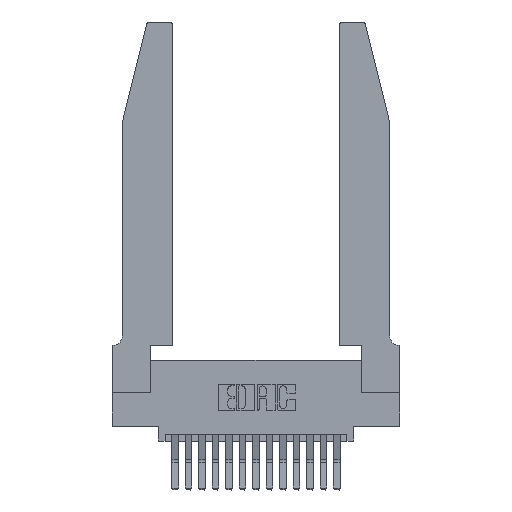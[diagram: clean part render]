
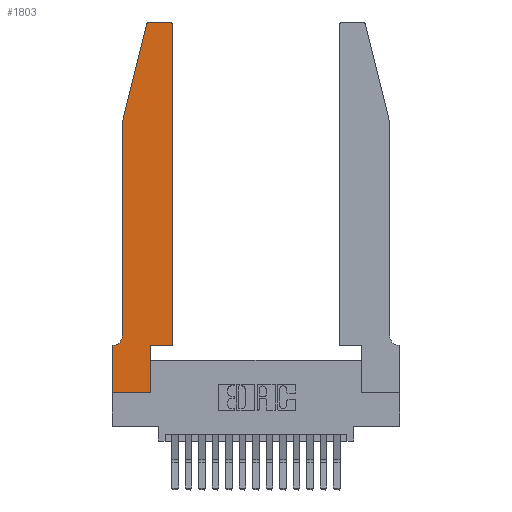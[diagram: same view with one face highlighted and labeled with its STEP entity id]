
A CAD part, top view. The second image highlights one B-rep face of the part: STEP entity #1803.
In plain terms, the highlighted planar face has unit normal (0, 0, 1).
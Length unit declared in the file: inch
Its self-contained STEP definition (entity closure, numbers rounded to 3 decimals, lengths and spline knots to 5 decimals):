
#357 = VERTEX_POINT ( 'NONE', #715 ) ;
#449 = AXIS2_PLACEMENT_3D ( 'NONE', #3735, #16731, #18242 ) ;
#673 = LINE ( 'NONE', #10025, #14673 ) ;
#715 = CARTESIAN_POINT ( 'NONE',  ( 0.2865, 0.35, 0.37 ) ) ;
#806 = CARTESIAN_POINT ( 'NONE',  ( 0.0055, 0.42, 0.37 ) ) ;
#818 = VECTOR ( 'NONE', #17683, 39.37008 ) ;
#869 = VECTOR ( 'NONE', #14858, 39.37008 ) ;
#1104 = ORIENTED_EDGE ( 'NONE', *, *, #1536, .T. ) ;
#1217 = VECTOR ( 'NONE', #18431, 39.37008 ) ;
#1273 = VERTEX_POINT ( 'NONE', #3354 ) ;
#1335 = EDGE_CURVE ( 'NONE', #11629, #10156, #16044, .T. ) ;
#1536 = EDGE_CURVE ( 'NONE', #2989, #9075, #16977, .T. ) ;
#1762 = EDGE_CURVE ( 'NONE', #1273, #7864, #10066, .T. ) ;
#1780 = EDGE_CURVE ( 'NONE', #9075, #6343, #16939, .T. ) ;
#1803 = ADVANCED_FACE ( 'NONE', ( #9216 ), #12288, .T. ) ;
#1937 = EDGE_CURVE ( 'NONE', #10156, #17461, #10199, .T. ) ;
#2416 = AXIS2_PLACEMENT_3D ( 'NONE', #15321, #6591, #6460 ) ;
#2774 = LINE ( 'NONE', #13495, #18003 ) ;
#2815 = DIRECTION ( 'NONE',  ( 1., 0., 0. ) ) ;
#2926 = CIRCLE ( 'NONE', #15723, 0.07 ) ;
#2989 = VERTEX_POINT ( 'NONE', #16043 ) ;
#3165 = CARTESIAN_POINT ( 'NONE',  ( 0.0755, 2., 0.37 ) ) ;
#3354 = CARTESIAN_POINT ( 'NONE',  ( 0.4505, 2.72, 0.37 ) ) ;
#3355 = CARTESIAN_POINT ( 'NONE',  ( 0.0055, 0.35, 0.37 ) ) ;
#3501 = VERTEX_POINT ( 'NONE', #12996 ) ;
#3607 = DIRECTION ( 'NONE',  ( 0., 0., -1. ) ) ;
#3735 = CARTESIAN_POINT ( 'NONE',  ( 0.4205, 2.72, 0.37 ) ) ;
#3738 = LINE ( 'NONE', #7984, #9475 ) ;
#4122 = EDGE_CURVE ( 'NONE', #6117, #2989, #13686, .T. ) ;
#4734 = DIRECTION ( 'NONE',  ( -0.239, -0.971, 0. ) ) ;
#5915 = CARTESIAN_POINT ( 'NONE',  ( 0.0755, 0.42, 0.37 ) ) ;
#6117 = VERTEX_POINT ( 'NONE', #3355 ) ;
#6247 = ORIENTED_EDGE ( 'NONE', *, *, #11947, .T. ) ;
#6343 = VERTEX_POINT ( 'NONE', #10061 ) ;
#6460 = DIRECTION ( 'NONE',  ( 1., 0., 0. ) ) ;
#6463 = AXIS2_PLACEMENT_3D ( 'NONE', #11657, #7205, #2815 ) ;
#6591 = DIRECTION ( 'NONE',  ( 0., 0., 1. ) ) ;
#7061 = ORIENTED_EDGE ( 'NONE', *, *, #7689, .T. ) ;
#7205 = DIRECTION ( 'NONE',  ( 0., 0., 1. ) ) ;
#7267 = CARTESIAN_POINT ( 'NONE',  ( 0.284, 2.75, 0.37 ) ) ;
#7689 = EDGE_CURVE ( 'NONE', #7703, #11629, #12498, .T. ) ;
#7703 = VERTEX_POINT ( 'NONE', #7267 ) ;
#7725 = VECTOR ( 'NONE', #17189, 39.37008 ) ;
#7864 = VERTEX_POINT ( 'NONE', #17652 ) ;
#7879 = EDGE_CURVE ( 'NONE', #6343, #357, #2774, .T. ) ;
#7931 = CARTESIAN_POINT ( 'NONE',  ( 0., 0., 0.37 ) ) ;
#7984 = CARTESIAN_POINT ( 'NONE',  ( 0.4505, 0.35, 0.37 ) ) ;
#8126 = CARTESIAN_POINT ( 'NONE',  ( 0.4505, 0.35, 0.37 ) ) ;
#9005 = CARTESIAN_POINT ( 'NONE',  ( 0., 0., 0.37 ) ) ;
#9075 = VERTEX_POINT ( 'NONE', #13056 ) ;
#9216 = FACE_OUTER_BOUND ( 'NONE', #15425, .T. ) ;
#9310 = ORIENTED_EDGE ( 'NONE', *, *, #16591, .T. ) ;
#9475 = VECTOR ( 'NONE', #16996, 39.37008 ) ;
#10025 = CARTESIAN_POINT ( 'NONE',  ( 0.2605, 2.75, 0.37 ) ) ;
#10061 = CARTESIAN_POINT ( 'NONE',  ( 0.2865, 0., 0.37 ) ) ;
#10066 = CIRCLE ( 'NONE', #449, 0.03 ) ;
#10156 = VERTEX_POINT ( 'NONE', #17405 ) ;
#10199 = LINE ( 'NONE', #14134, #7725 ) ;
#10365 = ORIENTED_EDGE ( 'NONE', *, *, #1762, .T. ) ;
#10880 = VECTOR ( 'NONE', #12409, 39.37008 ) ;
#10912 = ORIENTED_EDGE ( 'NONE', *, *, #1780, .T. ) ;
#11303 = LINE ( 'NONE', #8126, #1217 ) ;
#11583 = CARTESIAN_POINT ( 'NONE',  ( 0.0755, 0.35, 0.37 ) ) ;
#11629 = VERTEX_POINT ( 'NONE', #12693 ) ;
#11657 = CARTESIAN_POINT ( 'NONE',  ( 0.284, 2.72, 0.37 ) ) ;
#11947 = EDGE_CURVE ( 'NONE', #7864, #7703, #673, .T. ) ;
#12288 = PLANE ( 'NONE',  #2416 ) ;
#12409 = DIRECTION ( 'NONE',  ( 1., 0., 0. ) ) ;
#12498 = CIRCLE ( 'NONE', #6463, 0.03 ) ;
#12693 = CARTESIAN_POINT ( 'NONE',  ( 0.25487, 2.72718, 0.37 ) ) ;
#12740 = EDGE_CURVE ( 'NONE', #17461, #6117, #2926, .T. ) ;
#12996 = CARTESIAN_POINT ( 'NONE',  ( 0.4505, 0.35, 0.37 ) ) ;
#13056 = CARTESIAN_POINT ( 'NONE',  ( 0., 0., 0.37 ) ) ;
#13076 = ORIENTED_EDGE ( 'NONE', *, *, #7879, .T. ) ;
#13153 = ORIENTED_EDGE ( 'NONE', *, *, #12740, .T. ) ;
#13233 = DIRECTION ( 'NONE',  ( 0., 1., 0. ) ) ;
#13495 = CARTESIAN_POINT ( 'NONE',  ( 0.2865, 0.35, 0.37 ) ) ;
#13517 = VECTOR ( 'NONE', #4734, 39.37008 ) ;
#13686 = LINE ( 'NONE', #11583, #818 ) ;
#14002 = ORIENTED_EDGE ( 'NONE', *, *, #15268, .T. ) ;
#14134 = CARTESIAN_POINT ( 'NONE',  ( 0.0755, 2., 0.37 ) ) ;
#14673 = VECTOR ( 'NONE', #15811, 39.37008 ) ;
#14858 = DIRECTION ( 'NONE',  ( 0., -1., 0. ) ) ;
#15268 = EDGE_CURVE ( 'NONE', #3501, #1273, #3738, .T. ) ;
#15321 = CARTESIAN_POINT ( 'NONE',  ( 0., 0.35, 0.37 ) ) ;
#15398 = DIRECTION ( 'NONE',  ( -1., 0., 0. ) ) ;
#15425 = EDGE_LOOP ( 'NONE', ( #6247, #7061, #16685, #15951, #13153, #15449, #1104, #10912, #13076, #9310, #14002, #10365 ) ) ;
#15449 = ORIENTED_EDGE ( 'NONE', *, *, #4122, .T. ) ;
#15723 = AXIS2_PLACEMENT_3D ( 'NONE', #806, #3607, #15398 ) ;
#15811 = DIRECTION ( 'NONE',  ( -1., 0., 0. ) ) ;
#15951 = ORIENTED_EDGE ( 'NONE', *, *, #1937, .T. ) ;
#16043 = CARTESIAN_POINT ( 'NONE',  ( 0., 0.35, 0.37 ) ) ;
#16044 = LINE ( 'NONE', #3165, #13517 ) ;
#16591 = EDGE_CURVE ( 'NONE', #357, #3501, #11303, .T. ) ;
#16685 = ORIENTED_EDGE ( 'NONE', *, *, #1335, .T. ) ;
#16731 = DIRECTION ( 'NONE',  ( 0., 0., 1. ) ) ;
#16939 = LINE ( 'NONE', #7931, #10880 ) ;
#16977 = LINE ( 'NONE', #9005, #869 ) ;
#16996 = DIRECTION ( 'NONE',  ( 0., 1., 0. ) ) ;
#17189 = DIRECTION ( 'NONE',  ( 0., -1., 0. ) ) ;
#17405 = CARTESIAN_POINT ( 'NONE',  ( 0.0755, 2., 0.37 ) ) ;
#17461 = VERTEX_POINT ( 'NONE', #5915 ) ;
#17652 = CARTESIAN_POINT ( 'NONE',  ( 0.4205, 2.75, 0.37 ) ) ;
#17683 = DIRECTION ( 'NONE',  ( -1., 0., 0. ) ) ;
#18003 = VECTOR ( 'NONE', #13233, 39.37008 ) ;
#18242 = DIRECTION ( 'NONE',  ( 1., 0., 0. ) ) ;
#18431 = DIRECTION ( 'NONE',  ( 1., 0., 0. ) ) ;
